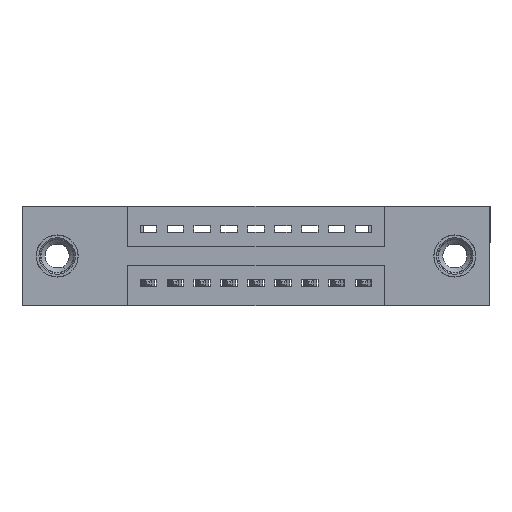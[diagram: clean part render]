
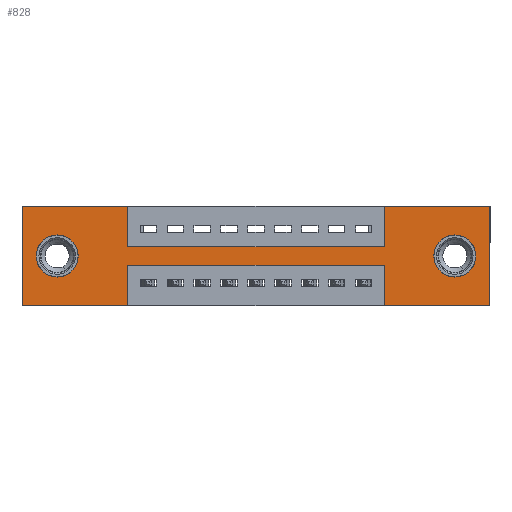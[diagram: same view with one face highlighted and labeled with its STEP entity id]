
A CAD part, front view. The second image highlights one B-rep face of the part: STEP entity #828.
In plain terms, the highlighted planar face has unit normal (0, -1, 0).
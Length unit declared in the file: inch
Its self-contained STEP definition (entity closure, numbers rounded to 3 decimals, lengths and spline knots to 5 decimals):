
#37 = AXIS2_PLACEMENT_3D ( 'NONE', #4863, #12179, #11013 ) ;
#43 = VERTEX_POINT ( 'NONE', #9777 ) ;
#498 = VECTOR ( 'NONE', #6706, 39.37008 ) ;
#623 = CARTESIAN_POINT ( 'NONE',  ( 1.735, 0., 0. ) ) ;
#828 = ADVANCED_FACE ( 'NONE', ( #13680, #14267, #10565 ), #5058, .T. ) ;
#855 = DIRECTION ( 'NONE',  ( 0., 0., 1. ) ) ;
#988 = CARTESIAN_POINT ( 'NONE',  ( 1.605, 0., -0.185 ) ) ;
#1023 = ORIENTED_EDGE ( 'NONE', *, *, #9639, .F. ) ;
#1227 = DIRECTION ( 'NONE',  ( -1., 0., 0. ) ) ;
#1239 = VERTEX_POINT ( 'NONE', #3948 ) ;
#1264 = CARTESIAN_POINT ( 'NONE',  ( 1.605, 0., -0.185 ) ) ;
#1293 = VERTEX_POINT ( 'NONE', #4162 ) ;
#1517 = CARTESIAN_POINT ( 'NONE',  ( 1.735, 0., 0. ) ) ;
#1581 = ORIENTED_EDGE ( 'NONE', *, *, #10109, .F. ) ;
#1626 = CIRCLE ( 'NONE', #11477, 0.078 ) ;
#1905 = EDGE_LOOP ( 'NONE', ( #12611, #3553 ) ) ;
#2042 = LINE ( 'NONE', #7999, #2402 ) ;
#2178 = VERTEX_POINT ( 'NONE', #8881 ) ;
#2191 = ORIENTED_EDGE ( 'NONE', *, *, #5368, .F. ) ;
#2306 = LINE ( 'NONE', #10714, #13300 ) ;
#2402 = VECTOR ( 'NONE', #14322, 39.37008 ) ;
#2730 = VECTOR ( 'NONE', #15901, 39.37008 ) ;
#2837 = CARTESIAN_POINT ( 'NONE',  ( 0., 0., -0.37 ) ) ;
#2864 = EDGE_CURVE ( 'NONE', #5402, #2178, #13173, .T. ) ;
#3071 = EDGE_CURVE ( 'NONE', #5095, #11120, #12208, .T. ) ;
#3111 = LINE ( 'NONE', #8224, #14868 ) ;
#3382 = VECTOR ( 'NONE', #15329, 39.37008 ) ;
#3505 = CARTESIAN_POINT ( 'NONE',  ( 0.13, 0., -0.107 ) ) ;
#3553 = ORIENTED_EDGE ( 'NONE', *, *, #14558, .T. ) ;
#3582 = LINE ( 'NONE', #623, #15005 ) ;
#3720 = LINE ( 'NONE', #5656, #498 ) ;
#3932 = DIRECTION ( 'NONE',  ( 0., 0., -1. ) ) ;
#3948 = CARTESIAN_POINT ( 'NONE',  ( 0., 0., 0. ) ) ;
#4162 = CARTESIAN_POINT ( 'NONE',  ( 1.735, 0., -0.37 ) ) ;
#4863 = CARTESIAN_POINT ( 'NONE',  ( 0.13, 0., -0.185 ) ) ;
#4870 = ORIENTED_EDGE ( 'NONE', *, *, #13713, .F. ) ;
#5058 = PLANE ( 'NONE',  #12781 ) ;
#5095 = VERTEX_POINT ( 'NONE', #9959 ) ;
#5291 = ORIENTED_EDGE ( 'NONE', *, *, #5999, .F. ) ;
#5353 = CARTESIAN_POINT ( 'NONE',  ( 1.3425, 0., -0.37 ) ) ;
#5356 = VERTEX_POINT ( 'NONE', #12589 ) ;
#5368 = EDGE_CURVE ( 'NONE', #8603, #43, #7073, .T. ) ;
#5402 = VERTEX_POINT ( 'NONE', #12127 ) ;
#5416 = AXIS2_PLACEMENT_3D ( 'NONE', #1264, #9975, #8742 ) ;
#5421 = EDGE_CURVE ( 'NONE', #6462, #14200, #11541, .T. ) ;
#5656 = CARTESIAN_POINT ( 'NONE',  ( 0., 0., -0.37 ) ) ;
#5689 = ORIENTED_EDGE ( 'NONE', *, *, #11371, .F. ) ;
#5727 = VECTOR ( 'NONE', #1227, 39.37008 ) ;
#5846 = ORIENTED_EDGE ( 'NONE', *, *, #6797, .F. ) ;
#5912 = CARTESIAN_POINT ( 'NONE',  ( 0., 0., 0. ) ) ;
#5999 = EDGE_CURVE ( 'NONE', #7928, #1293, #3582, .T. ) ;
#6075 = LINE ( 'NONE', #9844, #6474 ) ;
#6462 = VERTEX_POINT ( 'NONE', #10818 ) ;
#6474 = VECTOR ( 'NONE', #13592, 39.37008 ) ;
#6624 = ORIENTED_EDGE ( 'NONE', *, *, #8857, .F. ) ;
#6706 = DIRECTION ( 'NONE',  ( -1., 0., 0. ) ) ;
#6797 = EDGE_CURVE ( 'NONE', #14200, #8603, #6075, .T. ) ;
#6800 = ORIENTED_EDGE ( 'NONE', *, *, #5421, .F. ) ;
#7073 = LINE ( 'NONE', #2837, #11143 ) ;
#7233 = EDGE_CURVE ( 'NONE', #8362, #5356, #12258, .T. ) ;
#7540 = CIRCLE ( 'NONE', #8943, 0.078 ) ;
#7750 = DIRECTION ( 'NONE',  ( 0., 0., 1. ) ) ;
#7928 = VERTEX_POINT ( 'NONE', #1517 ) ;
#7999 = CARTESIAN_POINT ( 'NONE',  ( 0.3925, 0., 0. ) ) ;
#8020 = CARTESIAN_POINT ( 'NONE',  ( 0.3925, 0., -0.15 ) ) ;
#8224 = CARTESIAN_POINT ( 'NONE',  ( 0., 0., 0. ) ) ;
#8362 = VERTEX_POINT ( 'NONE', #3505 ) ;
#8368 = CARTESIAN_POINT ( 'NONE',  ( 0.3925, 0., 0. ) ) ;
#8566 = CARTESIAN_POINT ( 'NONE',  ( 1.605, 0., -0.263 ) ) ;
#8603 = VERTEX_POINT ( 'NONE', #15241 ) ;
#8742 = DIRECTION ( 'NONE',  ( 0., 0., -1. ) ) ;
#8857 = EDGE_CURVE ( 'NONE', #1239, #13796, #3111, .T. ) ;
#8881 = CARTESIAN_POINT ( 'NONE',  ( 1.3425, 0., 0. ) ) ;
#8943 = AXIS2_PLACEMENT_3D ( 'NONE', #988, #11927, #14461 ) ;
#9095 = VECTOR ( 'NONE', #11742, 39.37008 ) ;
#9238 = DIRECTION ( 'NONE',  ( 0., 0., -1. ) ) ;
#9267 = ORIENTED_EDGE ( 'NONE', *, *, #9430, .T. ) ;
#9284 = LINE ( 'NONE', #5912, #2730 ) ;
#9430 = EDGE_CURVE ( 'NONE', #11120, #5095, #7540, .T. ) ;
#9639 = EDGE_CURVE ( 'NONE', #12151, #6462, #11202, .T. ) ;
#9777 = CARTESIAN_POINT ( 'NONE',  ( 0., 0., -0.37 ) ) ;
#9844 = CARTESIAN_POINT ( 'NONE',  ( 0.3925, 0., -0.37 ) ) ;
#9959 = CARTESIAN_POINT ( 'NONE',  ( 1.605, 0., -0.107 ) ) ;
#9975 = DIRECTION ( 'NONE',  ( 0., 1., 0. ) ) ;
#10000 = ORIENTED_EDGE ( 'NONE', *, *, #13069, .F. ) ;
#10109 = EDGE_CURVE ( 'NONE', #2178, #7928, #9284, .T. ) ;
#10565 = FACE_OUTER_BOUND ( 'NONE', #12053, .T. ) ;
#10594 = ORIENTED_EDGE ( 'NONE', *, *, #2864, .F. ) ;
#10714 = CARTESIAN_POINT ( 'NONE',  ( 0., 0., 0. ) ) ;
#10818 = CARTESIAN_POINT ( 'NONE',  ( 1.3425, 0., -0.22 ) ) ;
#11013 = DIRECTION ( 'NONE',  ( 0., 0., 1. ) ) ;
#11120 = VERTEX_POINT ( 'NONE', #8566 ) ;
#11143 = VECTOR ( 'NONE', #15698, 39.37008 ) ;
#11202 = LINE ( 'NONE', #12830, #9095 ) ;
#11247 = ORIENTED_EDGE ( 'NONE', *, *, #13720, .F. ) ;
#11371 = EDGE_CURVE ( 'NONE', #43, #1239, #2306, .T. ) ;
#11477 = AXIS2_PLACEMENT_3D ( 'NONE', #12625, #13756, #7750 ) ;
#11493 = LINE ( 'NONE', #8020, #3382 ) ;
#11541 = LINE ( 'NONE', #15603, #5727 ) ;
#11742 = DIRECTION ( 'NONE',  ( 0., 0., 1. ) ) ;
#11748 = CARTESIAN_POINT ( 'NONE',  ( 1.3425, 0., 0. ) ) ;
#11927 = DIRECTION ( 'NONE',  ( 0., 1., 0. ) ) ;
#12053 = EDGE_LOOP ( 'NONE', ( #5846, #6800, #1023, #11247, #5291, #1581, #10594, #10000, #4870, #6624, #5689, #2191 ) ) ;
#12127 = CARTESIAN_POINT ( 'NONE',  ( 1.3425, 0., -0.15 ) ) ;
#12151 = VERTEX_POINT ( 'NONE', #5353 ) ;
#12179 = DIRECTION ( 'NONE',  ( 0., 1., 0. ) ) ;
#12208 = CIRCLE ( 'NONE', #5416, 0.078 ) ;
#12258 = CIRCLE ( 'NONE', #37, 0.078 ) ;
#12403 = VERTEX_POINT ( 'NONE', #12626 ) ;
#12589 = CARTESIAN_POINT ( 'NONE',  ( 0.13, 0., -0.263 ) ) ;
#12611 = ORIENTED_EDGE ( 'NONE', *, *, #7233, .T. ) ;
#12625 = CARTESIAN_POINT ( 'NONE',  ( 0.13, 0., -0.185 ) ) ;
#12626 = CARTESIAN_POINT ( 'NONE',  ( 0.3925, 0., -0.15 ) ) ;
#12781 = AXIS2_PLACEMENT_3D ( 'NONE', #13719, #14960, #3932 ) ;
#12830 = CARTESIAN_POINT ( 'NONE',  ( 1.3425, 0., -0.37 ) ) ;
#12859 = CARTESIAN_POINT ( 'NONE',  ( 0.3925, 0., -0.22 ) ) ;
#13069 = EDGE_CURVE ( 'NONE', #12403, #5402, #11493, .T. ) ;
#13173 = LINE ( 'NONE', #11748, #15290 ) ;
#13194 = DIRECTION ( 'NONE',  ( 0., 0., 1. ) ) ;
#13300 = VECTOR ( 'NONE', #13194, 39.37008 ) ;
#13592 = DIRECTION ( 'NONE',  ( 0., 0., -1. ) ) ;
#13680 = FACE_BOUND ( 'NONE', #13684, .T. ) ;
#13684 = EDGE_LOOP ( 'NONE', ( #15885, #9267 ) ) ;
#13713 = EDGE_CURVE ( 'NONE', #13796, #12403, #2042, .T. ) ;
#13719 = CARTESIAN_POINT ( 'NONE',  ( 0., 0., -0.37 ) ) ;
#13720 = EDGE_CURVE ( 'NONE', #1293, #12151, #3720, .T. ) ;
#13756 = DIRECTION ( 'NONE',  ( 0., 1., 0. ) ) ;
#13796 = VERTEX_POINT ( 'NONE', #8368 ) ;
#14200 = VERTEX_POINT ( 'NONE', #12859 ) ;
#14267 = FACE_BOUND ( 'NONE', #1905, .T. ) ;
#14322 = DIRECTION ( 'NONE',  ( 0., 0., -1. ) ) ;
#14461 = DIRECTION ( 'NONE',  ( 0., 0., -1. ) ) ;
#14558 = EDGE_CURVE ( 'NONE', #5356, #8362, #1626, .T. ) ;
#14868 = VECTOR ( 'NONE', #15802, 39.37008 ) ;
#14960 = DIRECTION ( 'NONE',  ( 0., -1., 0. ) ) ;
#15005 = VECTOR ( 'NONE', #9238, 39.37008 ) ;
#15241 = CARTESIAN_POINT ( 'NONE',  ( 0.3925, 0., -0.37 ) ) ;
#15290 = VECTOR ( 'NONE', #855, 39.37008 ) ;
#15329 = DIRECTION ( 'NONE',  ( 1., 0., 0. ) ) ;
#15603 = CARTESIAN_POINT ( 'NONE',  ( 0.3925, 0., -0.22 ) ) ;
#15698 = DIRECTION ( 'NONE',  ( -1., 0., 0. ) ) ;
#15802 = DIRECTION ( 'NONE',  ( 1., 0., 0. ) ) ;
#15885 = ORIENTED_EDGE ( 'NONE', *, *, #3071, .T. ) ;
#15901 = DIRECTION ( 'NONE',  ( 1., 0., 0. ) ) ;
